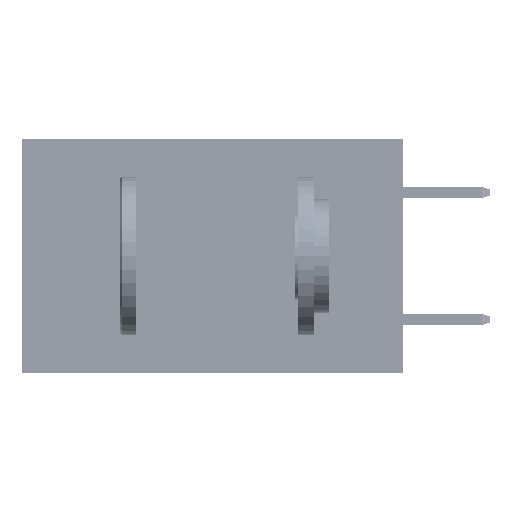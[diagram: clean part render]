
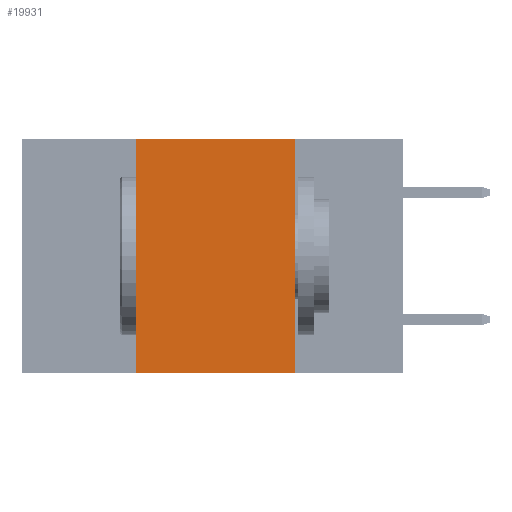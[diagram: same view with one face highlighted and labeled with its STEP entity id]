
A CAD part, left-side view. The second image highlights one B-rep face of the part: STEP entity #19931.
In plain terms, the highlighted planar face has unit normal (-1, 0, 0).
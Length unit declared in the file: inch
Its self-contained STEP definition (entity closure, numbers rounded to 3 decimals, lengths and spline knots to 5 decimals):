
#1430 = DIRECTION ( 'NONE',  ( 1., 0., 0. ) ) ;
#2063 = EDGE_CURVE ( 'NONE', #36289, #24748, #50845, .T. ) ;
#6264 = CARTESIAN_POINT ( 'NONE',  ( 0., 0.6, -0.37 ) ) ;
#9674 = CARTESIAN_POINT ( 'NONE',  ( 0., 0.42, 0. ) ) ;
#11295 = EDGE_CURVE ( 'NONE', #35922, #51508, #23848, .T. ) ;
#12558 = CARTESIAN_POINT ( 'NONE',  ( 0., 0.6, 0. ) ) ;
#12910 = EDGE_CURVE ( 'NONE', #36289, #35922, #19567, .T. ) ;
#14352 = LINE ( 'NONE', #38430, #36538 ) ;
#16003 = CARTESIAN_POINT ( 'NONE',  ( 0., 0.6, 0. ) ) ;
#16215 = ORIENTED_EDGE ( 'NONE', *, *, #11295, .F. ) ;
#16898 = VECTOR ( 'NONE', #24917, 39.37008 ) ;
#19567 = LINE ( 'NONE', #36069, #35174 ) ;
#19825 = ORIENTED_EDGE ( 'NONE', *, *, #2063, .T. ) ;
#19931 = ADVANCED_FACE ( 'NONE', ( #28512 ), #49602, .F. ) ;
#23848 = LINE ( 'NONE', #16003, #16898 ) ;
#24714 = ORIENTED_EDGE ( 'NONE', *, *, #38329, .F. ) ;
#24748 = VERTEX_POINT ( 'NONE', #47491 ) ;
#24917 = DIRECTION ( 'NONE',  ( 0., -1., 0. ) ) ;
#25116 = AXIS2_PLACEMENT_3D ( 'NONE', #12558, #1430, #42507 ) ;
#25728 = DIRECTION ( 'NONE',  ( 0., 0., -1. ) ) ;
#28512 = FACE_OUTER_BOUND ( 'NONE', #44022, .T. ) ;
#30782 = VECTOR ( 'NONE', #34915, 39.37008 ) ;
#34915 = DIRECTION ( 'NONE',  ( 0., -1., 0. ) ) ;
#35174 = VECTOR ( 'NONE', #52534, 39.37008 ) ;
#35922 = VERTEX_POINT ( 'NONE', #9674 ) ;
#36069 = CARTESIAN_POINT ( 'NONE',  ( 0., 0.42, 0. ) ) ;
#36289 = VERTEX_POINT ( 'NONE', #49355 ) ;
#36538 = VECTOR ( 'NONE', #25728, 39.37008 ) ;
#38329 = EDGE_CURVE ( 'NONE', #51508, #24748, #14352, .T. ) ;
#38430 = CARTESIAN_POINT ( 'NONE',  ( 0., 0.17, 0. ) ) ;
#42507 = DIRECTION ( 'NONE',  ( 0., 0., -1. ) ) ;
#44022 = EDGE_LOOP ( 'NONE', ( #24714, #16215, #46433, #19825 ) ) ;
#46433 = ORIENTED_EDGE ( 'NONE', *, *, #12910, .F. ) ;
#46712 = CARTESIAN_POINT ( 'NONE',  ( 0., 0.17, 0. ) ) ;
#47491 = CARTESIAN_POINT ( 'NONE',  ( 0., 0.17, -0.37 ) ) ;
#49355 = CARTESIAN_POINT ( 'NONE',  ( 0., 0.42, -0.37 ) ) ;
#49602 = PLANE ( 'NONE',  #25116 ) ;
#50845 = LINE ( 'NONE', #6264, #30782 ) ;
#51508 = VERTEX_POINT ( 'NONE', #46712 ) ;
#52534 = DIRECTION ( 'NONE',  ( 0., 0., 1. ) ) ;
